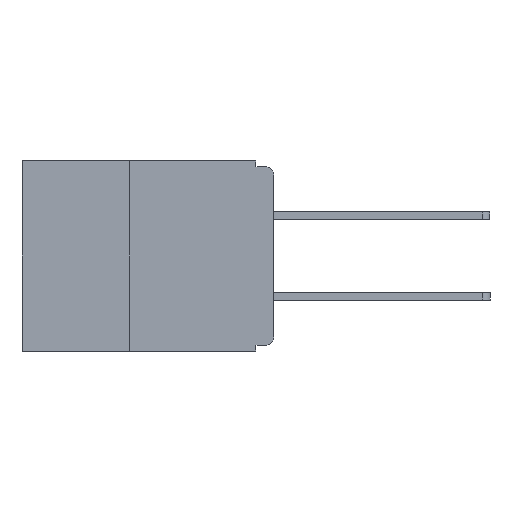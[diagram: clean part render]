
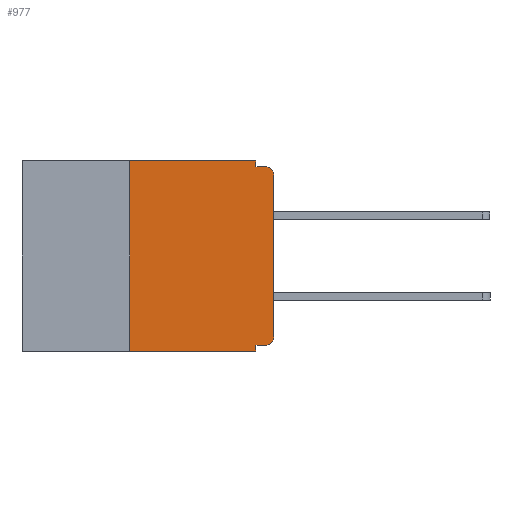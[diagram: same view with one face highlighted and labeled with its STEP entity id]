
A CAD part, left-side view. The second image highlights one B-rep face of the part: STEP entity #977.
In plain terms, the highlighted planar face has unit normal (-1, 0, 0).
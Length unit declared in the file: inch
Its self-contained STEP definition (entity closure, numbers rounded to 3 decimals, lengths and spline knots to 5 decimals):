
#40 = VERTEX_POINT ( 'NONE', #692 ) ;
#201 = ORIENTED_EDGE ( 'NONE', *, *, #7604, .T. ) ;
#552 = VECTOR ( 'NONE', #6463, 39.37008 ) ;
#553 = DIRECTION ( 'NONE',  ( 0., 0., 1. ) ) ;
#692 = CARTESIAN_POINT ( 'NONE',  ( 0., 0., -0.025 ) ) ;
#826 = DIRECTION ( 'NONE',  ( 0., 0., -1. ) ) ;
#875 = AXIS2_PLACEMENT_3D ( 'NONE', #7028, #6978, #826 ) ;
#977 = ADVANCED_FACE ( 'NONE', ( #8358 ), #13791, .F. ) ;
#1025 = EDGE_CURVE ( 'NONE', #40, #11502, #11122, .T. ) ;
#1498 = EDGE_CURVE ( 'NONE', #4840, #14663, #8001, .T. ) ;
#1617 = VECTOR ( 'NONE', #6019, 39.37008 ) ;
#1685 = VECTOR ( 'NONE', #4043, 39.37008 ) ;
#1896 = EDGE_CURVE ( 'NONE', #14954, #9098, #11808, .T. ) ;
#2081 = CARTESIAN_POINT ( 'NONE',  ( 0., 0.031, 0. ) ) ;
#2227 = EDGE_CURVE ( 'NONE', #8933, #11502, #10157, .T. ) ;
#2515 = ORIENTED_EDGE ( 'NONE', *, *, #7581, .F. ) ;
#2553 = AXIS2_PLACEMENT_3D ( 'NONE', #6657, #10312, #11314 ) ;
#4019 = DIRECTION ( 'NONE',  ( 0., 0., -1. ) ) ;
#4043 = DIRECTION ( 'NONE',  ( 0., 1., 0. ) ) ;
#4241 = ORIENTED_EDGE ( 'NONE', *, *, #1498, .F. ) ;
#4790 = CARTESIAN_POINT ( 'NONE',  ( 0., 0.437, 0. ) ) ;
#4792 = VECTOR ( 'NONE', #12555, 39.37008 ) ;
#4840 = VERTEX_POINT ( 'NONE', #13911 ) ;
#4933 = LINE ( 'NONE', #11148, #1685 ) ;
#4991 = ORIENTED_EDGE ( 'NONE', *, *, #1896, .T. ) ;
#5300 = EDGE_LOOP ( 'NONE', ( #15258, #7072, #10171, #2515, #15084, #11823, #201, #4241, #14012, #4991 ) ) ;
#5451 = CARTESIAN_POINT ( 'NONE',  ( 0., 0.25, 0. ) ) ;
#5821 = CARTESIAN_POINT ( 'NONE',  ( 0., 0., -0.305 ) ) ;
#5914 = EDGE_CURVE ( 'NONE', #9098, #40, #11729, .T. ) ;
#6019 = DIRECTION ( 'NONE',  ( 0., -1., 0. ) ) ;
#6022 = CARTESIAN_POINT ( 'NONE',  ( 0., 0.015, -0.305 ) ) ;
#6463 = DIRECTION ( 'NONE',  ( 0., -1., 0. ) ) ;
#6657 = CARTESIAN_POINT ( 'NONE',  ( 0., 0.015, -0.025 ) ) ;
#6978 = DIRECTION ( 'NONE',  ( 1., 0., 0. ) ) ;
#7028 = CARTESIAN_POINT ( 'NONE',  ( 0., 0.437, 0. ) ) ;
#7072 = ORIENTED_EDGE ( 'NONE', *, *, #1025, .T. ) ;
#7314 = VECTOR ( 'NONE', #4019, 39.37008 ) ;
#7554 = VERTEX_POINT ( 'NONE', #10856 ) ;
#7563 = DIRECTION ( 'NONE',  ( 0., 0., -1. ) ) ;
#7581 = EDGE_CURVE ( 'NONE', #14965, #8933, #10414, .T. ) ;
#7604 = EDGE_CURVE ( 'NONE', #7554, #14663, #13127, .T. ) ;
#8001 = LINE ( 'NONE', #12605, #4792 ) ;
#8346 = CARTESIAN_POINT ( 'NONE',  ( 0., 0.015, -0.01 ) ) ;
#8358 = FACE_OUTER_BOUND ( 'NONE', #5300, .T. ) ;
#8403 = LINE ( 'NONE', #4790, #1617 ) ;
#8738 = EDGE_CURVE ( 'NONE', #7554, #11393, #12750, .T. ) ;
#8933 = VERTEX_POINT ( 'NONE', #9081 ) ;
#9081 = CARTESIAN_POINT ( 'NONE',  ( 0., 0.031, -0.01 ) ) ;
#9089 = AXIS2_PLACEMENT_3D ( 'NONE', #6022, #9552, #7563 ) ;
#9098 = VERTEX_POINT ( 'NONE', #5821 ) ;
#9296 = VECTOR ( 'NONE', #14495, 39.37008 ) ;
#9430 = CARTESIAN_POINT ( 'NONE',  ( 0., 0., -0.01 ) ) ;
#9552 = DIRECTION ( 'NONE',  ( -1., 0., 0. ) ) ;
#10037 = VECTOR ( 'NONE', #14635, 39.37008 ) ;
#10157 = LINE ( 'NONE', #9430, #552 ) ;
#10171 = ORIENTED_EDGE ( 'NONE', *, *, #2227, .F. ) ;
#10312 = DIRECTION ( 'NONE',  ( -1., 0., 0. ) ) ;
#10414 = LINE ( 'NONE', #13178, #7314 ) ;
#10458 = CARTESIAN_POINT ( 'NONE',  ( 0., 0.015, -0.32 ) ) ;
#10614 = EDGE_CURVE ( 'NONE', #14954, #4840, #4933, .T. ) ;
#10856 = CARTESIAN_POINT ( 'NONE',  ( 0., 0.25, -0.33 ) ) ;
#11122 = CIRCLE ( 'NONE', #2553, 0.015 ) ;
#11148 = CARTESIAN_POINT ( 'NONE',  ( 0., 0., -0.32 ) ) ;
#11314 = DIRECTION ( 'NONE',  ( 0., 0., -1. ) ) ;
#11393 = VERTEX_POINT ( 'NONE', #5451 ) ;
#11502 = VERTEX_POINT ( 'NONE', #8346 ) ;
#11729 = LINE ( 'NONE', #13697, #14483 ) ;
#11808 = CIRCLE ( 'NONE', #9089, 0.015 ) ;
#11823 = ORIENTED_EDGE ( 'NONE', *, *, #8738, .F. ) ;
#12283 = CARTESIAN_POINT ( 'NONE',  ( 0., 0.437, -0.33 ) ) ;
#12555 = DIRECTION ( 'NONE',  ( 0., 0., -1. ) ) ;
#12605 = CARTESIAN_POINT ( 'NONE',  ( 0., 0.031, -0.33 ) ) ;
#12750 = LINE ( 'NONE', #14546, #9296 ) ;
#13127 = LINE ( 'NONE', #12283, #10037 ) ;
#13137 = CARTESIAN_POINT ( 'NONE',  ( 0., 0.031, -0.33 ) ) ;
#13178 = CARTESIAN_POINT ( 'NONE',  ( 0., 0.031, 0. ) ) ;
#13334 = EDGE_CURVE ( 'NONE', #11393, #14965, #8403, .T. ) ;
#13697 = CARTESIAN_POINT ( 'NONE',  ( 0., 0., 0. ) ) ;
#13791 = PLANE ( 'NONE',  #875 ) ;
#13911 = CARTESIAN_POINT ( 'NONE',  ( 0., 0.031, -0.32 ) ) ;
#14012 = ORIENTED_EDGE ( 'NONE', *, *, #10614, .F. ) ;
#14483 = VECTOR ( 'NONE', #553, 39.37008 ) ;
#14495 = DIRECTION ( 'NONE',  ( 0., 0., 1. ) ) ;
#14546 = CARTESIAN_POINT ( 'NONE',  ( 0., 0.25, -0.33 ) ) ;
#14635 = DIRECTION ( 'NONE',  ( 0., -1., 0. ) ) ;
#14663 = VERTEX_POINT ( 'NONE', #13137 ) ;
#14954 = VERTEX_POINT ( 'NONE', #10458 ) ;
#14965 = VERTEX_POINT ( 'NONE', #2081 ) ;
#15084 = ORIENTED_EDGE ( 'NONE', *, *, #13334, .F. ) ;
#15258 = ORIENTED_EDGE ( 'NONE', *, *, #5914, .T. ) ;
